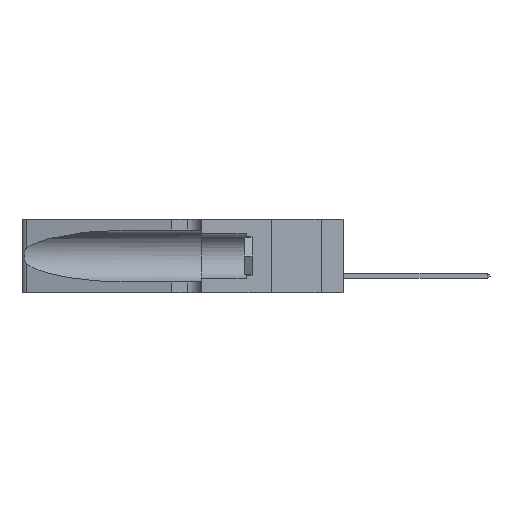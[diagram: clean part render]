
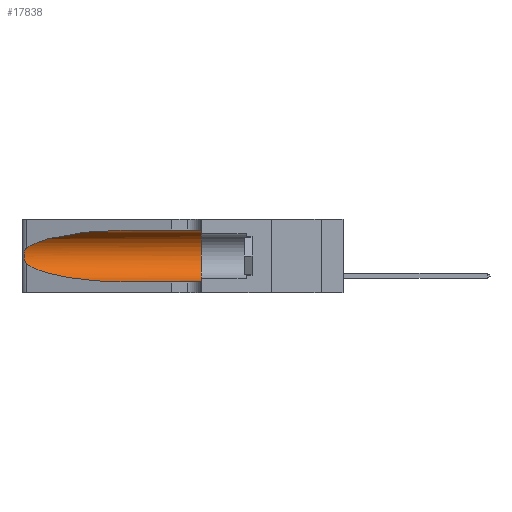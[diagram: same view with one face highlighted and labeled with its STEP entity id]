
A CAD part, left-side view. The second image highlights one B-rep face of the part: STEP entity #17838.
In plain terms, the highlighted cylindrical face has radius 3.308 mm (diameter 6.617 mm), a partial arc.
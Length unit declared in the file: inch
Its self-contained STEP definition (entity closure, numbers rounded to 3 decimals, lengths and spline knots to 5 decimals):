
#310 = EDGE_CURVE ( 'NONE', #12004, #22360, #28068, .T. ) ;
#943 = AXIS2_PLACEMENT_3D ( 'NONE', #21906, #30128, #24647 ) ;
#1769 = CARTESIAN_POINT ( 'NONE',  ( 0.25787, 1.23484, 0.2124 ) ) ;
#2005 = CARTESIAN_POINT ( 'NONE',  ( 0.25487, 1.22718, 0.14631 ) ) ;
#2194 = DIRECTION ( 'NONE',  ( 0., -1., 0. ) ) ;
#2230 = CARTESIAN_POINT ( 'NONE',  ( 0.25487, 1.22718, 0.22369 ) ) ;
#2245 = CARTESIAN_POINT ( 'NONE',  ( 0.25639, 1.23184, 0.21858 ) ) ;
#2896 = ORIENTED_EDGE ( 'NONE', *, *, #22727, .T. ) ;
#3154 = VECTOR ( 'NONE', #2194, 39.37008 ) ;
#3431 = DIRECTION ( 'NONE',  ( 0., -1., 0. ) ) ;
#3542 = DIRECTION ( 'NONE',  ( 0., 0., -1. ) ) ;
#3612 = EDGE_LOOP ( 'NONE', ( #25402, #2896, #20498, #11485, #21074, #7684 ) ) ;
#3698 = DIRECTION ( 'NONE',  ( 0., -1., 0. ) ) ;
#4028 = CARTESIAN_POINT ( 'NONE',  ( 0.25487, 1.22718, 0.14631 ) ) ;
#4436 = LINE ( 'NONE', #15670, #3154 ) ;
#4685 = CARTESIAN_POINT ( 'NONE',  ( 0.1305, 0.72297, 0.31525 ) ) ;
#5018 =( BOUNDED_CURVE ( )  B_SPLINE_CURVE ( 3, ( #4685, #18541, #29114, #2230 ),
 .UNSPECIFIED., .F., .F. ) 
 B_SPLINE_CURVE_WITH_KNOTS ( ( 4, 4 ),
 ( 1.5708, 2.84003 ),
 .UNSPECIFIED. ) 
 CURVE ( )  GEOMETRIC_REPRESENTATION_ITEM ( )  RATIONAL_B_SPLINE_CURVE ( ( 1., 0.87, 0.87, 1. ) ) 
 REPRESENTATION_ITEM ( '' )  );
#6287 = CARTESIAN_POINT ( 'NONE',  ( 0.1305, 0.72297, 0.05475 ) ) ;
#7684 = ORIENTED_EDGE ( 'NONE', *, *, #310, .F. ) ;
#8774 = CARTESIAN_POINT ( 'NONE',  ( 0.1305, 1.61858, 0.31525 ) ) ;
#9421 = CARTESIAN_POINT ( 'NONE',  ( 0.25487, 1.22718, 0.14631 ) ) ;
#11071 = CARTESIAN_POINT ( 'NONE',  ( 0.1305, 0.72297, 0.31525 ) ) ;
#11485 = ORIENTED_EDGE ( 'NONE', *, *, #19507, .T. ) ;
#12004 = VERTEX_POINT ( 'NONE', #11071 ) ;
#12482 = VERTEX_POINT ( 'NONE', #6287 ) ;
#12547 = AXIS2_PLACEMENT_3D ( 'NONE', #30222, #3431, #3542 ) ;
#12779 = CARTESIAN_POINT ( 'NONE',  ( 0.25555, 1.22994, 0.2215 ) ) ;
#12893 = CARTESIAN_POINT ( 'NONE',  ( 0.26075, 1.23896, 0.19203 ) ) ;
#14575 = VERTEX_POINT ( 'NONE', #4028 ) ;
#15328 = VECTOR ( 'NONE', #3698, 39.37008 ) ;
#15480 = CARTESIAN_POINT ( 'NONE',  ( 0.25854, 1.2359, 0.20912 ) ) ;
#15670 = CARTESIAN_POINT ( 'NONE',  ( 0.1305, 1.61858, 0.05475 ) ) ;
#15730 = CARTESIAN_POINT ( 'NONE',  ( 0.26018, 1.23835, 0.19895 ) ) ;
#15749 = VERTEX_POINT ( 'NONE', #21050 ) ;
#16796 = CARTESIAN_POINT ( 'NONE',  ( 0.1305, 0.35, 0.31525 ) ) ;
#17838 = ADVANCED_FACE ( 'NONE', ( #29578 ), #21488, .F. ) ;
#18440 = CARTESIAN_POINT ( 'NONE',  ( 0.25789, 1.23486, 0.15765 ) ) ;
#18541 = CARTESIAN_POINT ( 'NONE',  ( 0.18966, 0.96281, 0.31525 ) ) ;
#19151 = B_SPLINE_CURVE_WITH_KNOTS ( 'NONE', 3,
 ( #29013, #12779, #2245, #1769, #15480, #15730, #12893, #20696, #34722, #34490, #18440, #23421, #23884, #2005 ),
 .UNSPECIFIED., .F., .F.,
 ( 4, 2, 2, 2, 2, 2, 4 ),
 ( 0., 0.00027, 0.00053, 0.00107, 0.0016, 0.00187, 0.00214 ),
 .UNSPECIFIED. ) ;
#19507 = EDGE_CURVE ( 'NONE', #12482, #15749, #4436, .T. ) ;
#20498 = ORIENTED_EDGE ( 'NONE', *, *, #26244, .T. ) ;
#20696 = CARTESIAN_POINT ( 'NONE',  ( 0.26075, 1.23896, 0.178 ) ) ;
#21050 = CARTESIAN_POINT ( 'NONE',  ( 0.1305, 0.35, 0.05475 ) ) ;
#21074 = ORIENTED_EDGE ( 'NONE', *, *, #34759, .F. ) ;
#21488 = CYLINDRICAL_SURFACE ( 'NONE', #12547, 0.13025 ) ;
#21906 = CARTESIAN_POINT ( 'NONE',  ( 0.1305, 0.35, 0.185 ) ) ;
#22360 = VERTEX_POINT ( 'NONE', #16796 ) ;
#22414 = CARTESIAN_POINT ( 'NONE',  ( 0.18966, 0.96281, 0.05475 ) ) ;
#22727 = EDGE_CURVE ( 'NONE', #23445, #14575, #19151, .T. ) ;
#23421 = CARTESIAN_POINT ( 'NONE',  ( 0.25639, 1.23186, 0.15144 ) ) ;
#23445 = VERTEX_POINT ( 'NONE', #32414 ) ;
#23884 = CARTESIAN_POINT ( 'NONE',  ( 0.25555, 1.22993, 0.14849 ) ) ;
#24647 = DIRECTION ( 'NONE',  ( 0., 0., 1. ) ) ;
#25402 = ORIENTED_EDGE ( 'NONE', *, *, #32215, .T. ) ;
#25637 = CARTESIAN_POINT ( 'NONE',  ( 0.2373, 1.15595, 0.08982 ) ) ;
#26244 = EDGE_CURVE ( 'NONE', #14575, #12482, #30249, .T. ) ;
#28068 = LINE ( 'NONE', #8774, #15328 ) ;
#28381 = CARTESIAN_POINT ( 'NONE',  ( 0.1305, 0.72297, 0.05475 ) ) ;
#29013 = CARTESIAN_POINT ( 'NONE',  ( 0.25487, 1.22718, 0.22369 ) ) ;
#29114 = CARTESIAN_POINT ( 'NONE',  ( 0.2373, 1.15595, 0.28018 ) ) ;
#29578 = FACE_OUTER_BOUND ( 'NONE', #3612, .T. ) ;
#30128 = DIRECTION ( 'NONE',  ( 0., 1., 0. ) ) ;
#30222 = CARTESIAN_POINT ( 'NONE',  ( 0.1305, 1.61858, 0.185 ) ) ;
#30249 =( BOUNDED_CURVE ( )  B_SPLINE_CURVE ( 3, ( #9421, #25637, #22414, #28381 ),
 .UNSPECIFIED., .F., .F. ) 
 B_SPLINE_CURVE_WITH_KNOTS ( ( 4, 4 ),
 ( 3.44316, 4.71239 ),
 .UNSPECIFIED. ) 
 CURVE ( )  GEOMETRIC_REPRESENTATION_ITEM ( )  RATIONAL_B_SPLINE_CURVE ( ( 1., 0.87, 0.87, 1. ) ) 
 REPRESENTATION_ITEM ( '' )  );
#32215 = EDGE_CURVE ( 'NONE', #12004, #23445, #5018, .T. ) ;
#32414 = CARTESIAN_POINT ( 'NONE',  ( 0.25487, 1.22718, 0.22369 ) ) ;
#32606 = CIRCLE ( 'NONE', #943, 0.13025 ) ;
#34490 = CARTESIAN_POINT ( 'NONE',  ( 0.25856, 1.23593, 0.16098 ) ) ;
#34722 = CARTESIAN_POINT ( 'NONE',  ( 0.26017, 1.23833, 0.17102 ) ) ;
#34759 = EDGE_CURVE ( 'NONE', #22360, #15749, #32606, .T. ) ;
